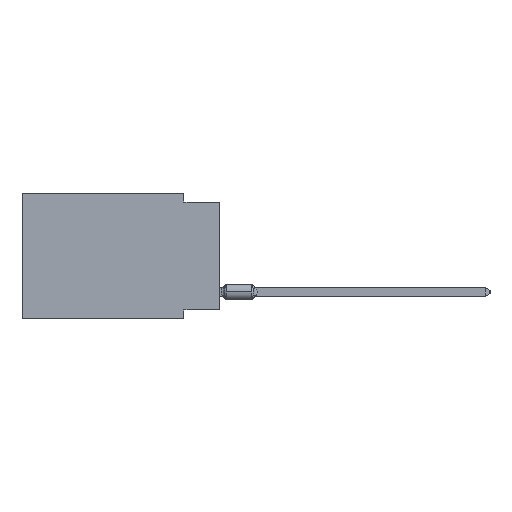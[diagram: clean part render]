
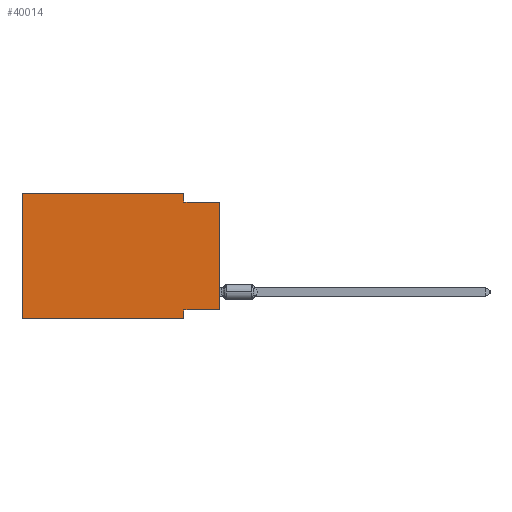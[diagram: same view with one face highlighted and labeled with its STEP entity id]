
A CAD part, left-side view. The second image highlights one B-rep face of the part: STEP entity #40014.
In plain terms, the highlighted planar face has unit normal (-1, 0, 0).
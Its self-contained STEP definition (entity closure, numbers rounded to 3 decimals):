
#1246 = ORIENTED_EDGE ( 'NONE', *, *, #18847, .F. ) ;
#2779 = VERTEX_POINT ( 'NONE', #59749 ) ;
#3250 = VERTEX_POINT ( 'NONE', #24594 ) ;
#3443 = ORIENTED_EDGE ( 'NONE', *, *, #40765, .F. ) ;
#3446 = VERTEX_POINT ( 'NONE', #64176 ) ;
#5019 = DIRECTION ( 'NONE',  ( 0., 1., 0. ) ) ;
#6946 = VERTEX_POINT ( 'NONE', #55205 ) ;
#7886 = EDGE_CURVE ( 'NONE', #13388, #3250, #28674, .T. ) ;
#10408 = CARTESIAN_POINT ( 'NONE',  ( 0., 13.97, 0. ) ) ;
#11393 = LINE ( 'NONE', #60048, #60414 ) ;
#13031 = VECTOR ( 'NONE', #57207, 1000. ) ;
#13388 = VERTEX_POINT ( 'NONE', #49932 ) ;
#13540 = DIRECTION ( 'NONE',  ( 0., -1., 0. ) ) ;
#15542 = EDGE_CURVE ( 'NONE', #51601, #2779, #34178, .T. ) ;
#16122 = DIRECTION ( 'NONE',  ( 0., 0., 1. ) ) ;
#17189 = LINE ( 'NONE', #52251, #44098 ) ;
#18362 = CARTESIAN_POINT ( 'NONE',  ( 0., 13.97, -8.89 ) ) ;
#18847 = EDGE_CURVE ( 'NONE', #3250, #44744, #11393, .T. ) ;
#19298 = PLANE ( 'NONE',  #19793 ) ;
#19793 = AXIS2_PLACEMENT_3D ( 'NONE', #59319, #41417, #53595 ) ;
#20829 = EDGE_CURVE ( 'NONE', #69423, #6946, #37813, .T. ) ;
#22371 = EDGE_CURVE ( 'NONE', #3446, #51601, #17189, .T. ) ;
#24026 = LINE ( 'NONE', #47269, #13031 ) ;
#24095 = DIRECTION ( 'NONE',  ( 0., -1., 0. ) ) ;
#24594 = CARTESIAN_POINT ( 'NONE',  ( 0., 13.97, 0. ) ) ;
#25008 = ORIENTED_EDGE ( 'NONE', *, *, #20829, .F. ) ;
#25113 = LINE ( 'NONE', #59797, #34415 ) ;
#28674 = LINE ( 'NONE', #10408, #35056 ) ;
#30925 = EDGE_LOOP ( 'NONE', ( #47130, #25008, #3443, #1246, #65556, #67839, #32708, #70925 ) ) ;
#31587 = DIRECTION ( 'NONE',  ( 0., 0., -1. ) ) ;
#32095 = DIRECTION ( 'NONE',  ( 0., -1., 0. ) ) ;
#32708 = ORIENTED_EDGE ( 'NONE', *, *, #15542, .F. ) ;
#34178 = LINE ( 'NONE', #51726, #38319 ) ;
#34415 = VECTOR ( 'NONE', #31587, 1000. ) ;
#35056 = VECTOR ( 'NONE', #16122, 1000. ) ;
#37813 = LINE ( 'NONE', #56463, #47403 ) ;
#38319 = VECTOR ( 'NONE', #46374, 1000. ) ;
#39296 = EDGE_CURVE ( 'NONE', #13388, #2779, #48839, .T. ) ;
#40014 = ADVANCED_FACE ( 'NONE', ( #72263 ), #19298, .F. ) ;
#40765 = EDGE_CURVE ( 'NONE', #44744, #69423, #25113, .T. ) ;
#41417 = DIRECTION ( 'NONE',  ( 1., 0., 0. ) ) ;
#44098 = VECTOR ( 'NONE', #5019, 1000. ) ;
#44744 = VERTEX_POINT ( 'NONE', #45601 ) ;
#45257 = VECTOR ( 'NONE', #24095, 1000. ) ;
#45601 = CARTESIAN_POINT ( 'NONE',  ( 0., 2.54, 0. ) ) ;
#46374 = DIRECTION ( 'NONE',  ( 0., 0., -1. ) ) ;
#47130 = ORIENTED_EDGE ( 'NONE', *, *, #54726, .T. ) ;
#47269 = CARTESIAN_POINT ( 'NONE',  ( 0., 0., 0. ) ) ;
#47403 = VECTOR ( 'NONE', #32095, 1000. ) ;
#48839 = LINE ( 'NONE', #18362, #45257 ) ;
#49932 = CARTESIAN_POINT ( 'NONE',  ( 0., 13.97, -8.89 ) ) ;
#51601 = VERTEX_POINT ( 'NONE', #62248 ) ;
#51726 = CARTESIAN_POINT ( 'NONE',  ( 0., 2.54, -8.89 ) ) ;
#52251 = CARTESIAN_POINT ( 'NONE',  ( 0., 0., -8.255 ) ) ;
#53595 = DIRECTION ( 'NONE',  ( 0., 0., -1. ) ) ;
#54726 = EDGE_CURVE ( 'NONE', #3446, #6946, #24026, .T. ) ;
#55205 = CARTESIAN_POINT ( 'NONE',  ( 0., 0., -0.635 ) ) ;
#56463 = CARTESIAN_POINT ( 'NONE',  ( 0., 0., -0.635 ) ) ;
#57207 = DIRECTION ( 'NONE',  ( 0., 0., 1. ) ) ;
#59319 = CARTESIAN_POINT ( 'NONE',  ( 0., 13.97, 0. ) ) ;
#59749 = CARTESIAN_POINT ( 'NONE',  ( 0., 2.54, -8.89 ) ) ;
#59797 = CARTESIAN_POINT ( 'NONE',  ( 0., 2.54, 0. ) ) ;
#60048 = CARTESIAN_POINT ( 'NONE',  ( 0., 13.97, 0. ) ) ;
#60414 = VECTOR ( 'NONE', #13540, 1000. ) ;
#62248 = CARTESIAN_POINT ( 'NONE',  ( 0., 2.54, -8.255 ) ) ;
#63470 = CARTESIAN_POINT ( 'NONE',  ( 0., 2.54, -0.635 ) ) ;
#64176 = CARTESIAN_POINT ( 'NONE',  ( 0., 0., -8.255 ) ) ;
#65556 = ORIENTED_EDGE ( 'NONE', *, *, #7886, .F. ) ;
#67839 = ORIENTED_EDGE ( 'NONE', *, *, #39296, .T. ) ;
#69423 = VERTEX_POINT ( 'NONE', #63470 ) ;
#70925 = ORIENTED_EDGE ( 'NONE', *, *, #22371, .F. ) ;
#72263 = FACE_OUTER_BOUND ( 'NONE', #30925, .T. ) ;
